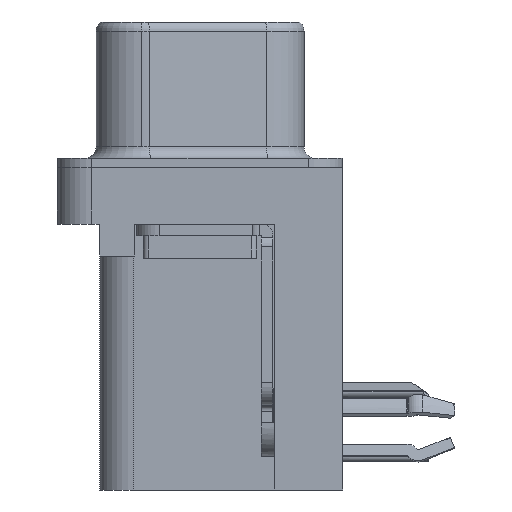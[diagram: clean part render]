
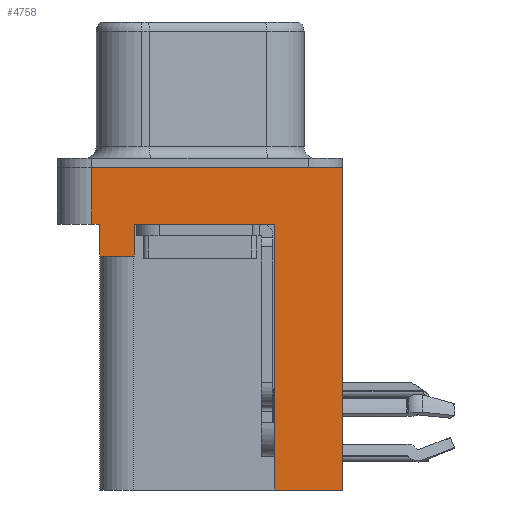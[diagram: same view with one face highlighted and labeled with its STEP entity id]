
A CAD part, left-side view. The second image highlights one B-rep face of the part: STEP entity #4758.
In plain terms, the highlighted planar face has unit normal (-1, 0, 0).
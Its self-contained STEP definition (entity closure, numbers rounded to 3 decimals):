
#55 = AXIS2_PLACEMENT_3D ( 'NONE', #2164, #5297, #6960 ) ;
#392 = EDGE_CURVE ( 'NONE', #9980, #4876, #14284, .T. ) ;
#602 = ORIENTED_EDGE ( 'NONE', *, *, #11805, .T. ) ;
#1347 = ORIENTED_EDGE ( 'NONE', *, *, #13295, .F. ) ;
#1374 = ORIENTED_EDGE ( 'NONE', *, *, #392, .F. ) ;
#1478 = EDGE_CURVE ( 'NONE', #21564, #5579, #3808, .T. ) ;
#1539 = VECTOR ( 'NONE', #15318, 1000. ) ;
#1825 = CARTESIAN_POINT ( 'NONE',  ( -3., 4.775, 0. ) ) ;
#2015 = DIRECTION ( 'NONE',  ( 0., -1., 0. ) ) ;
#2030 = DIRECTION ( 'NONE',  ( 0., 0., 1. ) ) ;
#2164 = CARTESIAN_POINT ( 'NONE',  ( -3., -6.275, -2.5 ) ) ;
#2227 = EDGE_CURVE ( 'NONE', #4876, #2946, #4320, .T. ) ;
#2908 = CARTESIAN_POINT ( 'NONE',  ( -3., -3.295, -2.5 ) ) ;
#2946 = VERTEX_POINT ( 'NONE', #4064 ) ;
#2997 = CARTESIAN_POINT ( 'NONE',  ( -3., -6.275, 0. ) ) ;
#3060 = CARTESIAN_POINT ( 'NONE',  ( -3., -6.275, -2.5 ) ) ;
#3145 = CARTESIAN_POINT ( 'NONE',  ( -3., 4.775, -2.5 ) ) ;
#3363 = VECTOR ( 'NONE', #16277, 1000. ) ;
#3470 = CARTESIAN_POINT ( 'NONE',  ( -3., -6.275, -2.5 ) ) ;
#3474 = CARTESIAN_POINT ( 'NONE',  ( -3., 2.895, -3.9 ) ) ;
#3613 = FACE_OUTER_BOUND ( 'NONE', #7040, .T. ) ;
#3646 = EDGE_CURVE ( 'NONE', #18246, #6033, #12550, .T. ) ;
#3808 = LINE ( 'NONE', #7143, #7964 ) ;
#3852 = CARTESIAN_POINT ( 'NONE',  ( -3., -6.275, -14.2 ) ) ;
#3975 = DIRECTION ( 'NONE',  ( 0., 0., 1. ) ) ;
#4012 = VECTOR ( 'NONE', #19424, 1000. ) ;
#4064 = CARTESIAN_POINT ( 'NONE',  ( -3., -6.275, 0. ) ) ;
#4091 = CARTESIAN_POINT ( 'NONE',  ( -3., 4.425, -3.9 ) ) ;
#4320 = LINE ( 'NONE', #2997, #3363 ) ;
#4389 = ORIENTED_EDGE ( 'NONE', *, *, #3646, .T. ) ;
#4758 = ADVANCED_FACE ( 'NONE', ( #3613 ), #7070, .T. ) ;
#4876 = VERTEX_POINT ( 'NONE', #1825 ) ;
#5297 = DIRECTION ( 'NONE',  ( -1., 0., 0. ) ) ;
#5379 = DIRECTION ( 'NONE',  ( 0., 1., 0. ) ) ;
#5405 = VERTEX_POINT ( 'NONE', #21013 ) ;
#5515 = ORIENTED_EDGE ( 'NONE', *, *, #1478, .F. ) ;
#5579 = VERTEX_POINT ( 'NONE', #2908 ) ;
#5720 = CARTESIAN_POINT ( 'NONE',  ( -3., 2.895, -3.9 ) ) ;
#5800 = CARTESIAN_POINT ( 'NONE',  ( -3., 4.775, -2.5 ) ) ;
#6033 = VERTEX_POINT ( 'NONE', #13378 ) ;
#6127 = VECTOR ( 'NONE', #18742, 1000. ) ;
#6868 = LINE ( 'NONE', #10442, #18445 ) ;
#6960 = DIRECTION ( 'NONE',  ( 0., 0., 1. ) ) ;
#7040 = EDGE_LOOP ( 'NONE', ( #20326, #1374, #602, #14100, #1347, #4389, #14028, #5515, #9627, #13697 ) ) ;
#7070 = PLANE ( 'NONE',  #55 ) ;
#7143 = CARTESIAN_POINT ( 'NONE',  ( -3., -3.295, -14.2 ) ) ;
#7585 = EDGE_CURVE ( 'NONE', #5405, #21580, #21181, .T. ) ;
#7964 = VECTOR ( 'NONE', #2030, 1000. ) ;
#8809 = LINE ( 'NONE', #15840, #6127 ) ;
#8963 = EDGE_CURVE ( 'NONE', #16013, #21564, #8809, .T. ) ;
#9627 = ORIENTED_EDGE ( 'NONE', *, *, #8963, .F. ) ;
#9761 = LINE ( 'NONE', #3060, #1539 ) ;
#9837 = CARTESIAN_POINT ( 'NONE',  ( -3., -3.295, -14.2 ) ) ;
#9980 = VERTEX_POINT ( 'NONE', #3145 ) ;
#10442 = CARTESIAN_POINT ( 'NONE',  ( -3., -6.275, -2.5 ) ) ;
#11805 = EDGE_CURVE ( 'NONE', #9980, #21580, #9761, .T. ) ;
#12416 = EDGE_CURVE ( 'NONE', #6033, #5579, #17304, .T. ) ;
#12550 = LINE ( 'NONE', #5720, #16382 ) ;
#13295 = EDGE_CURVE ( 'NONE', #18246, #5405, #15652, .T. ) ;
#13378 = CARTESIAN_POINT ( 'NONE',  ( -3., 2.895, -2.5 ) ) ;
#13686 = DIRECTION ( 'NONE',  ( 0., 0., 1. ) ) ;
#13697 = ORIENTED_EDGE ( 'NONE', *, *, #17312, .T. ) ;
#14028 = ORIENTED_EDGE ( 'NONE', *, *, #12416, .T. ) ;
#14100 = ORIENTED_EDGE ( 'NONE', *, *, #7585, .F. ) ;
#14284 = LINE ( 'NONE', #5800, #4012 ) ;
#14439 = VECTOR ( 'NONE', #5379, 1000. ) ;
#15318 = DIRECTION ( 'NONE',  ( 0., -1., 0. ) ) ;
#15652 = LINE ( 'NONE', #20689, #14439 ) ;
#15840 = CARTESIAN_POINT ( 'NONE',  ( -3., -3.295, -14.2 ) ) ;
#16013 = VERTEX_POINT ( 'NONE', #3852 ) ;
#16277 = DIRECTION ( 'NONE',  ( 0., -1., 0. ) ) ;
#16382 = VECTOR ( 'NONE', #17555, 1000. ) ;
#16648 = CARTESIAN_POINT ( 'NONE',  ( -3., 4.425, -2.5 ) ) ;
#17304 = LINE ( 'NONE', #3470, #19763 ) ;
#17312 = EDGE_CURVE ( 'NONE', #16013, #2946, #6868, .T. ) ;
#17319 = VECTOR ( 'NONE', #3975, 1000. ) ;
#17555 = DIRECTION ( 'NONE',  ( 0., 0., 1. ) ) ;
#18246 = VERTEX_POINT ( 'NONE', #3474 ) ;
#18445 = VECTOR ( 'NONE', #13686, 1000. ) ;
#18742 = DIRECTION ( 'NONE',  ( 0., 1., 0. ) ) ;
#19424 = DIRECTION ( 'NONE',  ( 0., 0., 1. ) ) ;
#19763 = VECTOR ( 'NONE', #2015, 1000. ) ;
#20326 = ORIENTED_EDGE ( 'NONE', *, *, #2227, .F. ) ;
#20689 = CARTESIAN_POINT ( 'NONE',  ( -3., 4.425, -3.9 ) ) ;
#21013 = CARTESIAN_POINT ( 'NONE',  ( -3., 4.425, -3.9 ) ) ;
#21181 = LINE ( 'NONE', #4091, #17319 ) ;
#21564 = VERTEX_POINT ( 'NONE', #9837 ) ;
#21580 = VERTEX_POINT ( 'NONE', #16648 ) ;
